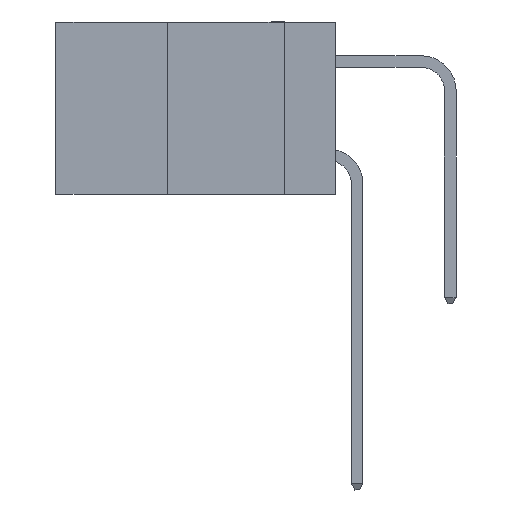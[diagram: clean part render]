
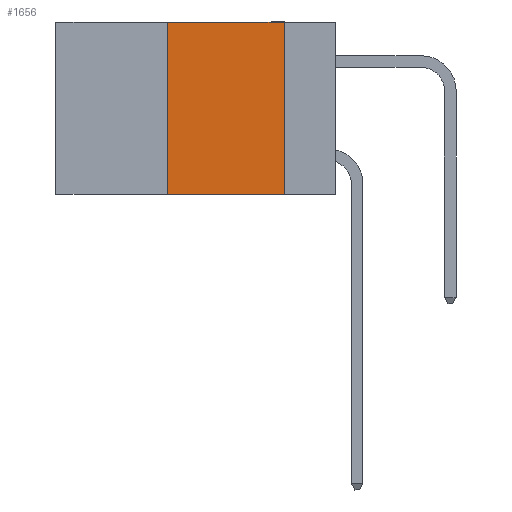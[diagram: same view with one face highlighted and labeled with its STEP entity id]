
A CAD part, left-side view. The second image highlights one B-rep face of the part: STEP entity #1656.
In plain terms, the highlighted planar face has unit normal (-1, 0, 0).
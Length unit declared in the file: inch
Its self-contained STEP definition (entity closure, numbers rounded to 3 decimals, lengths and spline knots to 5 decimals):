
#802 = VERTEX_POINT ( 'NONE', #6970 ) ;
#1085 = DIRECTION ( 'NONE',  ( 0., -1., 0. ) ) ;
#1105 = EDGE_CURVE ( 'NONE', #2709, #802, #11344, .T. ) ;
#1656 = ADVANCED_FACE ( 'NONE', ( #22899 ), #21896, .F. ) ;
#2709 = VERTEX_POINT ( 'NONE', #16658 ) ;
#3795 = CARTESIAN_POINT ( 'NONE',  ( 0., 0.11, 0. ) ) ;
#5516 = VECTOR ( 'NONE', #10702, 39.37008 ) ;
#5974 = CARTESIAN_POINT ( 'NONE',  ( 0., 0.36, 0. ) ) ;
#6970 = CARTESIAN_POINT ( 'NONE',  ( 0., 0.36, 0. ) ) ;
#7188 = CARTESIAN_POINT ( 'NONE',  ( 0., 0.11, -0.37 ) ) ;
#7305 = EDGE_CURVE ( 'NONE', #2709, #19689, #17979, .T. ) ;
#8093 = CARTESIAN_POINT ( 'NONE',  ( 0., 0.11, 0. ) ) ;
#8197 = EDGE_CURVE ( 'NONE', #802, #20326, #19567, .T. ) ;
#8290 = ORIENTED_EDGE ( 'NONE', *, *, #14879, .F. ) ;
#8595 = ORIENTED_EDGE ( 'NONE', *, *, #7305, .T. ) ;
#8715 = VECTOR ( 'NONE', #1085, 39.37008 ) ;
#9227 = ORIENTED_EDGE ( 'NONE', *, *, #1105, .F. ) ;
#10418 = DIRECTION ( 'NONE',  ( 1., 0., 0. ) ) ;
#10702 = DIRECTION ( 'NONE',  ( 0., -1., 0. ) ) ;
#11344 = LINE ( 'NONE', #5974, #15375 ) ;
#12360 = EDGE_LOOP ( 'NONE', ( #8290, #15184, #9227, #8595 ) ) ;
#13751 = CARTESIAN_POINT ( 'NONE',  ( 0., 0.6, -0.37 ) ) ;
#14157 = DIRECTION ( 'NONE',  ( 0., 0., -1. ) ) ;
#14863 = VECTOR ( 'NONE', #20295, 39.37008 ) ;
#14879 = EDGE_CURVE ( 'NONE', #20326, #19689, #18910, .T. ) ;
#15184 = ORIENTED_EDGE ( 'NONE', *, *, #8197, .F. ) ;
#15375 = VECTOR ( 'NONE', #22339, 39.37008 ) ;
#16658 = CARTESIAN_POINT ( 'NONE',  ( 0., 0.36, -0.37 ) ) ;
#16742 = AXIS2_PLACEMENT_3D ( 'NONE', #20767, #10418, #14157 ) ;
#17979 = LINE ( 'NONE', #13751, #8715 ) ;
#18910 = LINE ( 'NONE', #8093, #14863 ) ;
#19567 = LINE ( 'NONE', #21024, #5516 ) ;
#19689 = VERTEX_POINT ( 'NONE', #7188 ) ;
#20295 = DIRECTION ( 'NONE',  ( 0., 0., -1. ) ) ;
#20326 = VERTEX_POINT ( 'NONE', #3795 ) ;
#20767 = CARTESIAN_POINT ( 'NONE',  ( 0., 0.6, 0. ) ) ;
#21024 = CARTESIAN_POINT ( 'NONE',  ( 0., 0.6, 0. ) ) ;
#21896 = PLANE ( 'NONE',  #16742 ) ;
#22339 = DIRECTION ( 'NONE',  ( 0., 0., 1. ) ) ;
#22899 = FACE_OUTER_BOUND ( 'NONE', #12360, .T. ) ;
